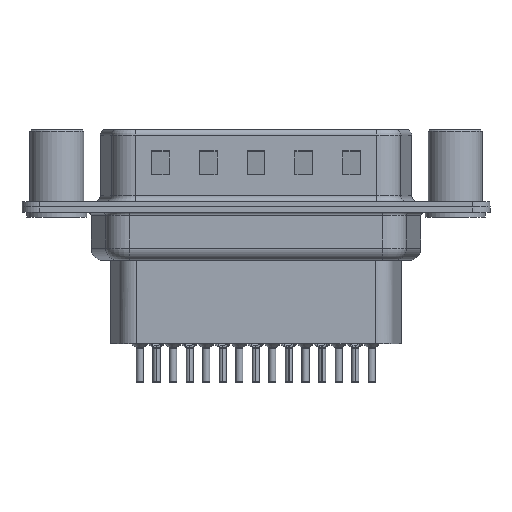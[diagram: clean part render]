
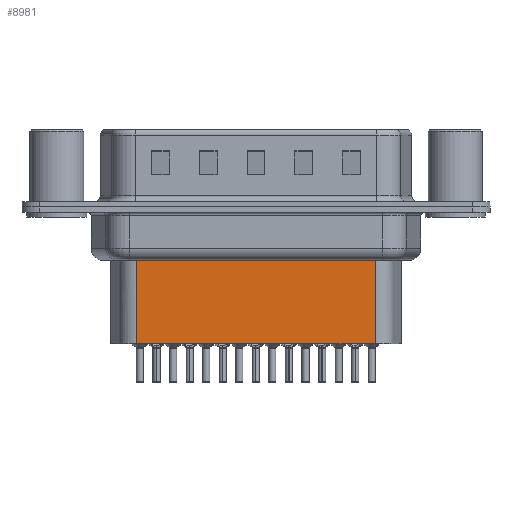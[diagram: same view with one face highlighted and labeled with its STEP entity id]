
A CAD part, front view. The second image highlights one B-rep face of the part: STEP entity #8981.
In plain terms, the highlighted planar face has unit normal (0, -1, 0).
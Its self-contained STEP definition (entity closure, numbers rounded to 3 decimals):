
#84 = VERTEX_POINT ( 'NONE', #5384 ) ;
#209 = EDGE_CURVE ( 'NONE', #84, #21366, #2259, .T. ) ;
#1709 = FACE_OUTER_BOUND ( 'NONE', #13006, .T. ) ;
#2025 = VECTOR ( 'NONE', #14235, 1000. ) ;
#2259 = LINE ( 'NONE', #4040, #6907 ) ;
#2364 = CARTESIAN_POINT ( 'NONE',  ( 6.681, -3.5, -11.45 ) ) ;
#2831 = ORIENTED_EDGE ( 'NONE', *, *, #20247, .F. ) ;
#3844 = EDGE_CURVE ( 'NONE', #12778, #12569, #17252, .T. ) ;
#4040 = CARTESIAN_POINT ( 'NONE',  ( 6.681, -3.5, -3.1 ) ) ;
#5123 = DIRECTION ( 'NONE',  ( 1., 0., 0. ) ) ;
#5384 = CARTESIAN_POINT ( 'NONE',  ( 6.681, -3.5, -4.097 ) ) ;
#6226 = ORIENTED_EDGE ( 'NONE', *, *, #7822, .T. ) ;
#6907 = VECTOR ( 'NONE', #16799, 1000. ) ;
#7822 = EDGE_CURVE ( 'NONE', #12778, #84, #11957, .T. ) ;
#8321 = DIRECTION ( 'NONE',  ( -1., 0., 0. ) ) ;
#8538 = CARTESIAN_POINT ( 'NONE',  ( 6.681, -3.5, -11.45 ) ) ;
#8789 = CARTESIAN_POINT ( 'NONE',  ( 26.619, -3.5, -4.097 ) ) ;
#8981 = ADVANCED_FACE ( 'NONE', ( #1709 ), #13508, .T. ) ;
#9824 = CARTESIAN_POINT ( 'NONE',  ( 26.619, -3.5, -11.45 ) ) ;
#11580 = ORIENTED_EDGE ( 'NONE', *, *, #3844, .F. ) ;
#11957 = LINE ( 'NONE', #14906, #19776 ) ;
#12569 = VERTEX_POINT ( 'NONE', #9824 ) ;
#12778 = VERTEX_POINT ( 'NONE', #8789 ) ;
#12848 = VECTOR ( 'NONE', #16551, 1000. ) ;
#13006 = EDGE_LOOP ( 'NONE', ( #11580, #6226, #20803, #2831 ) ) ;
#13508 = PLANE ( 'NONE',  #19816 ) ;
#14235 = DIRECTION ( 'NONE',  ( -1., 0., 0. ) ) ;
#14906 = CARTESIAN_POINT ( 'NONE',  ( 6.434, -3.5, -4.097 ) ) ;
#15002 = CARTESIAN_POINT ( 'NONE',  ( 6.681, -3.5, -3.1 ) ) ;
#15151 = DIRECTION ( 'NONE',  ( 0., -1., 0. ) ) ;
#15183 = CARTESIAN_POINT ( 'NONE',  ( 26.619, -3.5, -3.1 ) ) ;
#15536 = LINE ( 'NONE', #2364, #2025 ) ;
#16551 = DIRECTION ( 'NONE',  ( 0., 0., -1. ) ) ;
#16799 = DIRECTION ( 'NONE',  ( 0., 0., -1. ) ) ;
#17252 = LINE ( 'NONE', #15183, #12848 ) ;
#19776 = VECTOR ( 'NONE', #8321, 1000. ) ;
#19816 = AXIS2_PLACEMENT_3D ( 'NONE', #15002, #15151, #5123 ) ;
#20247 = EDGE_CURVE ( 'NONE', #12569, #21366, #15536, .T. ) ;
#20803 = ORIENTED_EDGE ( 'NONE', *, *, #209, .T. ) ;
#21366 = VERTEX_POINT ( 'NONE', #8538 ) ;
